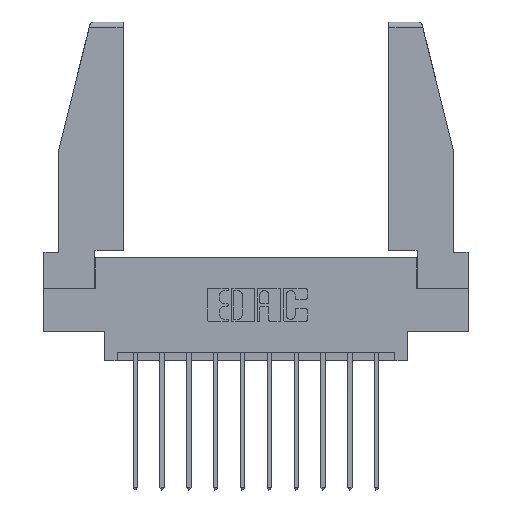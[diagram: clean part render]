
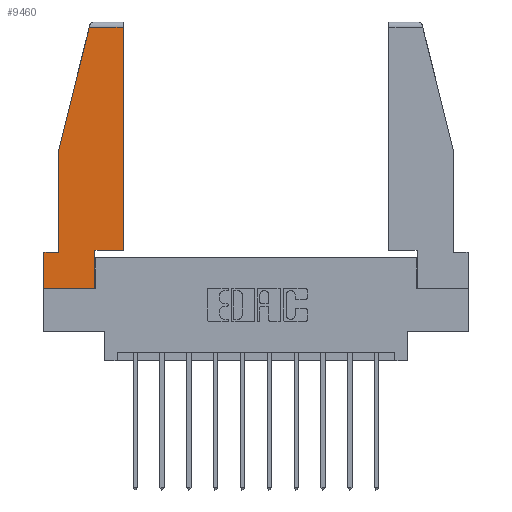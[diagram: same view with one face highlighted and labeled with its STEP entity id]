
A CAD part, top view. The second image highlights one B-rep face of the part: STEP entity #9460.
In plain terms, the highlighted planar face has unit normal (0, 0, 1).
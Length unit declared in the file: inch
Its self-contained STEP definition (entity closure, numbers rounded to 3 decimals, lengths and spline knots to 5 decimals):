
#24 = DIRECTION ( 'NONE',  ( 0., -1., 0. ) ) ;
#213 = CARTESIAN_POINT ( 'NONE',  ( 0., 0.21, 0. ) ) ;
#250 = VERTEX_POINT ( 'NONE', #3037 ) ;
#252 = CARTESIAN_POINT ( 'NONE',  ( 0.297, 0., 0. ) ) ;
#824 = VERTEX_POINT ( 'NONE', #11833 ) ;
#1070 = FACE_OUTER_BOUND ( 'NONE', #14173, .T. ) ;
#1138 = LINE ( 'NONE', #213, #6605 ) ;
#1458 = CARTESIAN_POINT ( 'NONE',  ( 0., 0.21, 0. ) ) ;
#1707 = EDGE_CURVE ( 'NONE', #5367, #13718, #13773, .T. ) ;
#1757 = EDGE_CURVE ( 'NONE', #7824, #5367, #1138, .T. ) ;
#1810 = CARTESIAN_POINT ( 'NONE',  ( 0., 0., 0. ) ) ;
#2152 = LINE ( 'NONE', #1458, #7456 ) ;
#2183 = ORIENTED_EDGE ( 'NONE', *, *, #1757, .T. ) ;
#2501 = CARTESIAN_POINT ( 'NONE',  ( 0.271, 1.55, 0. ) ) ;
#2552 = DIRECTION ( 'NONE',  ( -0.239, -0.971, 0. ) ) ;
#2687 = EDGE_CURVE ( 'NONE', #14099, #250, #4081, .T. ) ;
#2727 = EDGE_CURVE ( 'NONE', #824, #7824, #2152, .T. ) ;
#2860 = VECTOR ( 'NONE', #10117, 39.37008 ) ;
#2863 = ORIENTED_EDGE ( 'NONE', *, *, #1707, .T. ) ;
#3037 = CARTESIAN_POINT ( 'NONE',  ( 0.2636, 1.52, 0. ) ) ;
#3090 = EDGE_CURVE ( 'NONE', #12827, #14099, #12340, .T. ) ;
#3382 = EDGE_CURVE ( 'NONE', #13830, #12827, #10931, .T. ) ;
#3642 = EDGE_CURVE ( 'NONE', #250, #9585, #10751, .T. ) ;
#3764 = CARTESIAN_POINT ( 'NONE',  ( 0., 0., 0. ) ) ;
#3850 = DIRECTION ( 'NONE',  ( 0., -1., 0. ) ) ;
#3860 = DIRECTION ( 'NONE',  ( -1., 0., 0. ) ) ;
#3917 = CARTESIAN_POINT ( 'NONE',  ( 0.086, 0.8, 0. ) ) ;
#4081 = LINE ( 'NONE', #5775, #9526 ) ;
#4144 = AXIS2_PLACEMENT_3D ( 'NONE', #3764, #6068, #12732 ) ;
#4474 = VECTOR ( 'NONE', #12379, 39.37008 ) ;
#4544 = CARTESIAN_POINT ( 'NONE',  ( 0., 0., 0. ) ) ;
#4566 = VECTOR ( 'NONE', #8519, 39.37008 ) ;
#5367 = VERTEX_POINT ( 'NONE', #1810 ) ;
#5457 = ORIENTED_EDGE ( 'NONE', *, *, #12441, .T. ) ;
#5775 = CARTESIAN_POINT ( 'NONE',  ( 0., 1.52, 0. ) ) ;
#5823 = LINE ( 'NONE', #9472, #4566 ) ;
#6068 = DIRECTION ( 'NONE',  ( 0., 0., 1. ) ) ;
#6277 = CARTESIAN_POINT ( 'NONE',  ( 0.297, 0.223, 0. ) ) ;
#6605 = VECTOR ( 'NONE', #24, 39.37008 ) ;
#7093 = EDGE_CURVE ( 'NONE', #13718, #13830, #5823, .T. ) ;
#7340 = CARTESIAN_POINT ( 'NONE',  ( 0.461, 1.52, 0. ) ) ;
#7377 = PLANE ( 'NONE',  #4144 ) ;
#7456 = VECTOR ( 'NONE', #3860, 39.37008 ) ;
#7824 = VERTEX_POINT ( 'NONE', #9620 ) ;
#8129 = CARTESIAN_POINT ( 'NONE',  ( 0.086, 0.8, 0. ) ) ;
#8280 = ORIENTED_EDGE ( 'NONE', *, *, #3382, .T. ) ;
#8394 = ORIENTED_EDGE ( 'NONE', *, *, #3090, .T. ) ;
#8519 = DIRECTION ( 'NONE',  ( 0., 1., 0. ) ) ;
#9071 = DIRECTION ( 'NONE',  ( -1., 0., 0. ) ) ;
#9183 = VECTOR ( 'NONE', #2552, 39.37008 ) ;
#9343 = ORIENTED_EDGE ( 'NONE', *, *, #2687, .T. ) ;
#9344 = VECTOR ( 'NONE', #9711, 39.37008 ) ;
#9460 = ADVANCED_FACE ( 'NONE', ( #1070 ), #7377, .T. ) ;
#9472 = CARTESIAN_POINT ( 'NONE',  ( 0.297, 0., 0. ) ) ;
#9526 = VECTOR ( 'NONE', #9071, 39.37008 ) ;
#9585 = VERTEX_POINT ( 'NONE', #3917 ) ;
#9620 = CARTESIAN_POINT ( 'NONE',  ( 0., 0.21, 0. ) ) ;
#9711 = DIRECTION ( 'NONE',  ( 1., 0., 0. ) ) ;
#10117 = DIRECTION ( 'NONE',  ( 0., 1., 0. ) ) ;
#10692 = CARTESIAN_POINT ( 'NONE',  ( 0.461, 0.223, 0. ) ) ;
#10751 = LINE ( 'NONE', #2501, #9183 ) ;
#10931 = LINE ( 'NONE', #6277, #9344 ) ;
#11241 = ORIENTED_EDGE ( 'NONE', *, *, #3642, .T. ) ;
#11736 = CARTESIAN_POINT ( 'NONE',  ( 0.297, 0.223, 0. ) ) ;
#11833 = CARTESIAN_POINT ( 'NONE',  ( 0.086, 0.21, 0. ) ) ;
#12029 = ORIENTED_EDGE ( 'NONE', *, *, #7093, .T. ) ;
#12248 = ORIENTED_EDGE ( 'NONE', *, *, #2727, .T. ) ;
#12340 = LINE ( 'NONE', #13708, #2860 ) ;
#12379 = DIRECTION ( 'NONE',  ( 1., 0., 0. ) ) ;
#12441 = EDGE_CURVE ( 'NONE', #9585, #824, #13562, .T. ) ;
#12732 = DIRECTION ( 'NONE',  ( 1., 0., 0. ) ) ;
#12827 = VERTEX_POINT ( 'NONE', #10692 ) ;
#13391 = VECTOR ( 'NONE', #3850, 39.37008 ) ;
#13562 = LINE ( 'NONE', #8129, #13391 ) ;
#13708 = CARTESIAN_POINT ( 'NONE',  ( 0.461, 0.223, 0. ) ) ;
#13718 = VERTEX_POINT ( 'NONE', #252 ) ;
#13773 = LINE ( 'NONE', #4544, #4474 ) ;
#13830 = VERTEX_POINT ( 'NONE', #11736 ) ;
#14099 = VERTEX_POINT ( 'NONE', #7340 ) ;
#14173 = EDGE_LOOP ( 'NONE', ( #8394, #9343, #11241, #5457, #12248, #2183, #2863, #12029, #8280 ) ) ;
